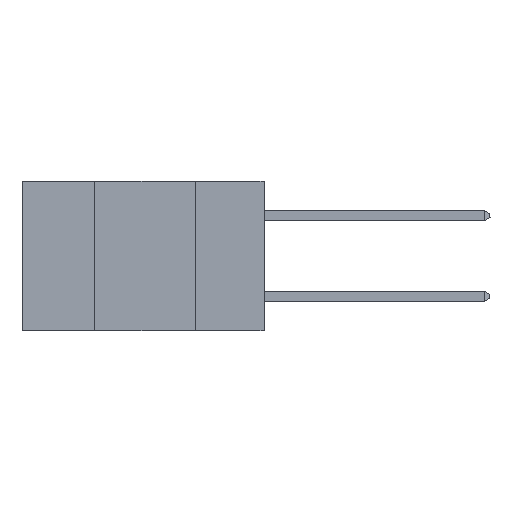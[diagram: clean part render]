
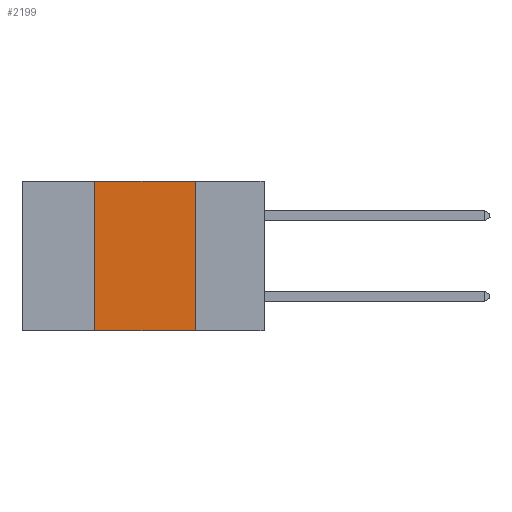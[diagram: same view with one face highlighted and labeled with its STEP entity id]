
A CAD part, left-side view. The second image highlights one B-rep face of the part: STEP entity #2199.
In plain terms, the highlighted planar face has unit normal (-1, 0, 0).
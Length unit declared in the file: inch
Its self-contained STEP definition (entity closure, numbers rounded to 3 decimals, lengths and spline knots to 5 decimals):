
#96 = VECTOR ( 'NONE', #3192, 39.37008 ) ;
#501 = CARTESIAN_POINT ( 'NONE',  ( 0., 0.42, 0. ) ) ;
#519 = CARTESIAN_POINT ( 'NONE',  ( 0., 0.42, 0. ) ) ;
#718 = VERTEX_POINT ( 'NONE', #1769 ) ;
#1437 = EDGE_CURVE ( 'NONE', #2357, #718, #11906, .T. ) ;
#1769 = CARTESIAN_POINT ( 'NONE',  ( 0., 0.17, -0.37 ) ) ;
#1875 = DIRECTION ( 'NONE',  ( 1., 0., 0. ) ) ;
#2199 = ADVANCED_FACE ( 'NONE', ( #6305 ), #7495, .F. ) ;
#2357 = VERTEX_POINT ( 'NONE', #3204 ) ;
#2563 = CARTESIAN_POINT ( 'NONE',  ( 0., 0.42, -0.37 ) ) ;
#2729 = DIRECTION ( 'NONE',  ( 0., 0., 1. ) ) ;
#3192 = DIRECTION ( 'NONE',  ( 0., -1., 0. ) ) ;
#3204 = CARTESIAN_POINT ( 'NONE',  ( 0., 0.17, 0. ) ) ;
#3544 = VERTEX_POINT ( 'NONE', #519 ) ;
#5011 = EDGE_CURVE ( 'NONE', #7287, #718, #9811, .T. ) ;
#5265 = ORIENTED_EDGE ( 'NONE', *, *, #10816, .F. ) ;
#5819 = VECTOR ( 'NONE', #9463, 39.37008 ) ;
#5838 = EDGE_LOOP ( 'NONE', ( #5903, #5923, #5265, #13408 ) ) ;
#5890 = EDGE_CURVE ( 'NONE', #3544, #2357, #11373, .T. ) ;
#5903 = ORIENTED_EDGE ( 'NONE', *, *, #1437, .F. ) ;
#5923 = ORIENTED_EDGE ( 'NONE', *, *, #5890, .F. ) ;
#6122 = VECTOR ( 'NONE', #9167, 39.37008 ) ;
#6305 = FACE_OUTER_BOUND ( 'NONE', #5838, .T. ) ;
#7287 = VERTEX_POINT ( 'NONE', #2563 ) ;
#7495 = PLANE ( 'NONE',  #8895 ) ;
#8624 = CARTESIAN_POINT ( 'NONE',  ( 0., 0.6, 0. ) ) ;
#8828 = DIRECTION ( 'NONE',  ( 0., 0., -1. ) ) ;
#8895 = AXIS2_PLACEMENT_3D ( 'NONE', #8624, #1875, #8828 ) ;
#9004 = LINE ( 'NONE', #501, #14220 ) ;
#9167 = DIRECTION ( 'NONE',  ( 0., -1., 0. ) ) ;
#9212 = CARTESIAN_POINT ( 'NONE',  ( 0., 0.6, 0. ) ) ;
#9463 = DIRECTION ( 'NONE',  ( 0., 0., -1. ) ) ;
#9811 = LINE ( 'NONE', #14377, #96 ) ;
#10816 = EDGE_CURVE ( 'NONE', #7287, #3544, #9004, .T. ) ;
#11373 = LINE ( 'NONE', #9212, #6122 ) ;
#11906 = LINE ( 'NONE', #13793, #5819 ) ;
#13408 = ORIENTED_EDGE ( 'NONE', *, *, #5011, .T. ) ;
#13793 = CARTESIAN_POINT ( 'NONE',  ( 0., 0.17, 0. ) ) ;
#14220 = VECTOR ( 'NONE', #2729, 39.37008 ) ;
#14377 = CARTESIAN_POINT ( 'NONE',  ( 0., 0.6, -0.37 ) ) ;
